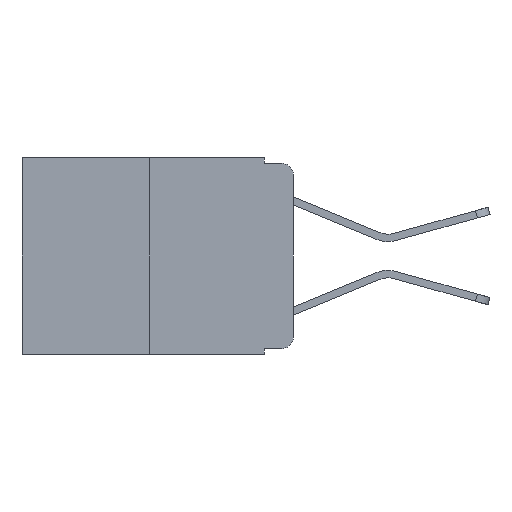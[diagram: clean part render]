
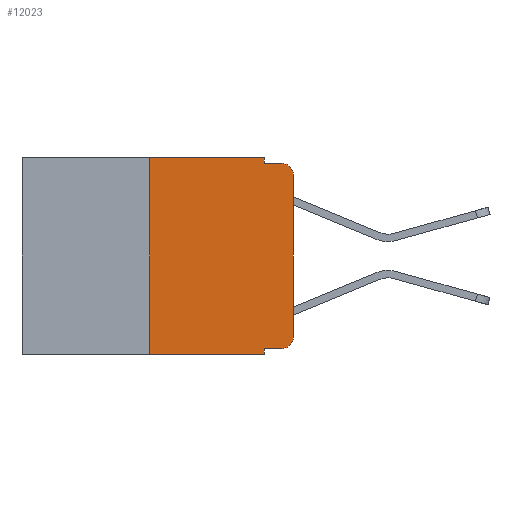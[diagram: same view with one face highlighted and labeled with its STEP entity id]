
A CAD part, left-side view. The second image highlights one B-rep face of the part: STEP entity #12023.
In plain terms, the highlighted planar face has unit normal (-1, 0, 0).
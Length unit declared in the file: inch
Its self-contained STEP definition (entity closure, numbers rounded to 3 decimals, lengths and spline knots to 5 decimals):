
#23 = CARTESIAN_POINT ( 'NONE',  ( 0., 0.25, 0. ) ) ;
#113 = DIRECTION ( 'NONE',  ( 1., 0., 0. ) ) ;
#557 = DIRECTION ( 'NONE',  ( 0., -1., 0. ) ) ;
#683 = LINE ( 'NONE', #8145, #6755 ) ;
#866 = VERTEX_POINT ( 'NONE', #13912 ) ;
#1046 = EDGE_CURVE ( 'NONE', #4919, #7831, #12951, .T. ) ;
#1296 = VECTOR ( 'NONE', #7693, 39.37008 ) ;
#1438 = VECTOR ( 'NONE', #3278, 39.37008 ) ;
#1583 = EDGE_CURVE ( 'NONE', #5849, #12903, #2791, .T. ) ;
#1638 = EDGE_CURVE ( 'NONE', #12903, #11448, #7735, .T. ) ;
#1663 = EDGE_CURVE ( 'NONE', #1870, #11448, #683, .T. ) ;
#1697 = EDGE_CURVE ( 'NONE', #866, #1870, #3372, .T. ) ;
#1756 = EDGE_CURVE ( 'NONE', #4919, #13644, #7576, .T. ) ;
#1835 = CARTESIAN_POINT ( 'NONE',  ( 0., 0.02, -0.01 ) ) ;
#1870 = VERTEX_POINT ( 'NONE', #11676 ) ;
#2374 = ORIENTED_EDGE ( 'NONE', *, *, #1046, .T. ) ;
#2435 = CARTESIAN_POINT ( 'NONE',  ( 0., 0.051, -0.333 ) ) ;
#2718 = LINE ( 'NONE', #4366, #13144 ) ;
#2791 = LINE ( 'NONE', #12313, #5912 ) ;
#2918 = DIRECTION ( 'NONE',  ( 0., -1., 0. ) ) ;
#3278 = DIRECTION ( 'NONE',  ( 0., -1., 0. ) ) ;
#3372 = LINE ( 'NONE', #12514, #8516 ) ;
#3641 = DIRECTION ( 'NONE',  ( -1., 0., 0. ) ) ;
#4178 = FACE_OUTER_BOUND ( 'NONE', #10471, .T. ) ;
#4366 = CARTESIAN_POINT ( 'NONE',  ( 0., 0.051, 0. ) ) ;
#4919 = VERTEX_POINT ( 'NONE', #6337 ) ;
#5186 = CARTESIAN_POINT ( 'NONE',  ( 0., 0.02, -0.03 ) ) ;
#5189 = ORIENTED_EDGE ( 'NONE', *, *, #1756, .F. ) ;
#5301 = AXIS2_PLACEMENT_3D ( 'NONE', #7311, #113, #8368 ) ;
#5414 = VECTOR ( 'NONE', #2918, 39.37008 ) ;
#5513 = EDGE_CURVE ( 'NONE', #6586, #7831, #2718, .T. ) ;
#5555 = DIRECTION ( 'NONE',  ( 0., 0., -1. ) ) ;
#5620 = EDGE_CURVE ( 'NONE', #6586, #13011, #12571, .T. ) ;
#5753 = LINE ( 'NONE', #8418, #5414 ) ;
#5819 = EDGE_CURVE ( 'NONE', #13011, #5849, #12998, .T. ) ;
#5849 = VERTEX_POINT ( 'NONE', #10036 ) ;
#5877 = CARTESIAN_POINT ( 'NONE',  ( 0., 0.25, 0. ) ) ;
#5912 = VECTOR ( 'NONE', #6367, 39.37008 ) ;
#6337 = CARTESIAN_POINT ( 'NONE',  ( 0., 0.25, -0.343 ) ) ;
#6367 = DIRECTION ( 'NONE',  ( 0., 0., 1. ) ) ;
#6378 = CARTESIAN_POINT ( 'NONE',  ( 0., 0.02, -0.333 ) ) ;
#6546 = DIRECTION ( 'NONE',  ( 0., 0., -1. ) ) ;
#6586 = VERTEX_POINT ( 'NONE', #2435 ) ;
#6755 = VECTOR ( 'NONE', #9657, 39.37008 ) ;
#6860 = ORIENTED_EDGE ( 'NONE', *, *, #1638, .T. ) ;
#7252 = CARTESIAN_POINT ( 'NONE',  ( 0., 0., -0.03 ) ) ;
#7311 = CARTESIAN_POINT ( 'NONE',  ( 0., 0.473, 0. ) ) ;
#7362 = PLANE ( 'NONE',  #5301 ) ;
#7576 = LINE ( 'NONE', #5877, #1296 ) ;
#7693 = DIRECTION ( 'NONE',  ( 0., 0., 1. ) ) ;
#7735 = CIRCLE ( 'NONE', #13829, 0.02 ) ;
#7831 = VERTEX_POINT ( 'NONE', #12973 ) ;
#7993 = DIRECTION ( 'NONE',  ( 0., 0., -1. ) ) ;
#8136 = ORIENTED_EDGE ( 'NONE', *, *, #1583, .T. ) ;
#8145 = CARTESIAN_POINT ( 'NONE',  ( 0., 0.051, -0.01 ) ) ;
#8368 = DIRECTION ( 'NONE',  ( 0., 0., -1. ) ) ;
#8418 = CARTESIAN_POINT ( 'NONE',  ( 0., 0.473, 0. ) ) ;
#8516 = VECTOR ( 'NONE', #5555, 39.37008 ) ;
#9657 = DIRECTION ( 'NONE',  ( 0., -1., 0. ) ) ;
#9712 = CARTESIAN_POINT ( 'NONE',  ( 0., 0.051, -0.333 ) ) ;
#9837 = EDGE_CURVE ( 'NONE', #13644, #866, #5753, .T. ) ;
#9998 = CARTESIAN_POINT ( 'NONE',  ( 0., 0.02, -0.313 ) ) ;
#10036 = CARTESIAN_POINT ( 'NONE',  ( 0., 0., -0.313 ) ) ;
#10331 = ORIENTED_EDGE ( 'NONE', *, *, #5513, .F. ) ;
#10375 = VECTOR ( 'NONE', #557, 39.37008 ) ;
#10471 = EDGE_LOOP ( 'NONE', ( #8136, #6860, #13324, #13934, #13039, #5189, #2374, #10331, #12010, #10652 ) ) ;
#10652 = ORIENTED_EDGE ( 'NONE', *, *, #5819, .T. ) ;
#10966 = DIRECTION ( 'NONE',  ( 0., 0., -1. ) ) ;
#11445 = DIRECTION ( 'NONE',  ( -1., 0., 0. ) ) ;
#11448 = VERTEX_POINT ( 'NONE', #1835 ) ;
#11676 = CARTESIAN_POINT ( 'NONE',  ( 0., 0.051, -0.01 ) ) ;
#12010 = ORIENTED_EDGE ( 'NONE', *, *, #5620, .T. ) ;
#12023 = ADVANCED_FACE ( 'NONE', ( #4178 ), #7362, .F. ) ;
#12313 = CARTESIAN_POINT ( 'NONE',  ( 0., 0., 0. ) ) ;
#12514 = CARTESIAN_POINT ( 'NONE',  ( 0., 0.051, 0. ) ) ;
#12571 = LINE ( 'NONE', #9712, #1438 ) ;
#12903 = VERTEX_POINT ( 'NONE', #7252 ) ;
#12951 = LINE ( 'NONE', #13306, #10375 ) ;
#12973 = CARTESIAN_POINT ( 'NONE',  ( 0., 0.051, -0.343 ) ) ;
#12998 = CIRCLE ( 'NONE', #14014, 0.02 ) ;
#13011 = VERTEX_POINT ( 'NONE', #6378 ) ;
#13039 = ORIENTED_EDGE ( 'NONE', *, *, #9837, .F. ) ;
#13144 = VECTOR ( 'NONE', #6546, 39.37008 ) ;
#13306 = CARTESIAN_POINT ( 'NONE',  ( 0., 0.473, -0.343 ) ) ;
#13324 = ORIENTED_EDGE ( 'NONE', *, *, #1663, .F. ) ;
#13644 = VERTEX_POINT ( 'NONE', #23 ) ;
#13829 = AXIS2_PLACEMENT_3D ( 'NONE', #5186, #11445, #7993 ) ;
#13912 = CARTESIAN_POINT ( 'NONE',  ( 0., 0.051, 0. ) ) ;
#13934 = ORIENTED_EDGE ( 'NONE', *, *, #1697, .F. ) ;
#14014 = AXIS2_PLACEMENT_3D ( 'NONE', #9998, #3641, #10966 ) ;
